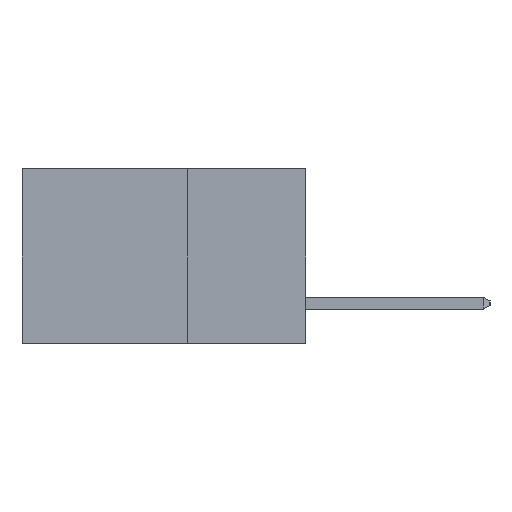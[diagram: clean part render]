
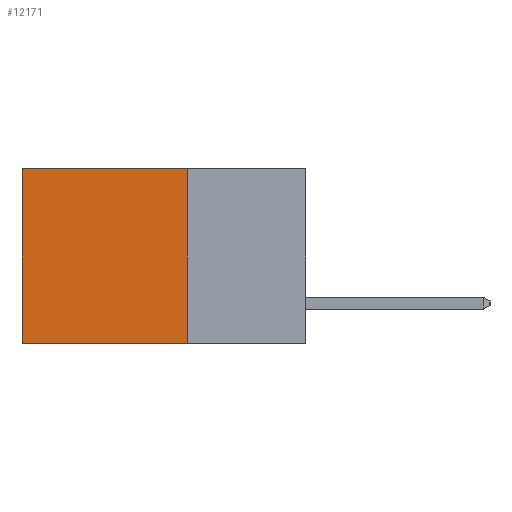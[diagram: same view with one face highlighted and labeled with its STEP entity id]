
A CAD part, left-side view. The second image highlights one B-rep face of the part: STEP entity #12171.
In plain terms, the highlighted planar face has unit normal (-1, 0, 0).
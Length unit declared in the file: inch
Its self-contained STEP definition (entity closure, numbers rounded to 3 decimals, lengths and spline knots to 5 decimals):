
#354 = VERTEX_POINT ( 'NONE', #6200 ) ;
#438 = VECTOR ( 'NONE', #9277, 39.37008 ) ;
#487 = EDGE_CURVE ( 'NONE', #1950, #354, #11210, .T. ) ;
#844 = CARTESIAN_POINT ( 'NONE',  ( 0.2615, 0.25, -0.37 ) ) ;
#1014 = CARTESIAN_POINT ( 'NONE',  ( 0.2615, 0.25, 0. ) ) ;
#1084 = CARTESIAN_POINT ( 'NONE',  ( 0.2615, 0.25, -0.37 ) ) ;
#1096 = PLANE ( 'NONE',  #13896 ) ;
#1950 = VERTEX_POINT ( 'NONE', #3942 ) ;
#2256 = EDGE_LOOP ( 'NONE', ( #2902, #6266, #12173, #14373 ) ) ;
#2902 = ORIENTED_EDGE ( 'NONE', *, *, #487, .T. ) ;
#3450 = DIRECTION ( 'NONE',  ( 0., 0., -1. ) ) ;
#3942 = CARTESIAN_POINT ( 'NONE',  ( 0.2615, 0.6, 0. ) ) ;
#4228 = CARTESIAN_POINT ( 'NONE',  ( 0.2615, 0.25, 0. ) ) ;
#4399 = CARTESIAN_POINT ( 'NONE',  ( 0.2615, 0.6, -0.37 ) ) ;
#4695 = CARTESIAN_POINT ( 'NONE',  ( 0.2615, 0.25, -0.37 ) ) ;
#5360 = VERTEX_POINT ( 'NONE', #844 ) ;
#5375 = DIRECTION ( 'NONE',  ( 0., 1., 0. ) ) ;
#5461 = FACE_OUTER_BOUND ( 'NONE', #2256, .T. ) ;
#5789 = VECTOR ( 'NONE', #11077, 39.37008 ) ;
#5862 = DIRECTION ( 'NONE',  ( 0., 1., 0. ) ) ;
#6008 = LINE ( 'NONE', #4228, #11788 ) ;
#6200 = CARTESIAN_POINT ( 'NONE',  ( 0.2615, 0.6, -0.37 ) ) ;
#6266 = ORIENTED_EDGE ( 'NONE', *, *, #6548, .F. ) ;
#6374 = LINE ( 'NONE', #4695, #12172 ) ;
#6548 = EDGE_CURVE ( 'NONE', #5360, #354, #6374, .T. ) ;
#8143 = EDGE_CURVE ( 'NONE', #13336, #1950, #6008, .T. ) ;
#9277 = DIRECTION ( 'NONE',  ( 0., 0., -1. ) ) ;
#9287 = CARTESIAN_POINT ( 'NONE',  ( 0.2615, 0.25, -0.37 ) ) ;
#9793 = LINE ( 'NONE', #1084, #438 ) ;
#10433 = DIRECTION ( 'NONE',  ( 1., 0., 0. ) ) ;
#11077 = DIRECTION ( 'NONE',  ( 0., 0., -1. ) ) ;
#11210 = LINE ( 'NONE', #4399, #5789 ) ;
#11788 = VECTOR ( 'NONE', #5375, 39.37008 ) ;
#12171 = ADVANCED_FACE ( 'NONE', ( #5461 ), #1096, .F. ) ;
#12172 = VECTOR ( 'NONE', #5862, 39.37008 ) ;
#12173 = ORIENTED_EDGE ( 'NONE', *, *, #12691, .F. ) ;
#12691 = EDGE_CURVE ( 'NONE', #13336, #5360, #9793, .T. ) ;
#13336 = VERTEX_POINT ( 'NONE', #1014 ) ;
#13896 = AXIS2_PLACEMENT_3D ( 'NONE', #9287, #10433, #3450 ) ;
#14373 = ORIENTED_EDGE ( 'NONE', *, *, #8143, .T. ) ;
